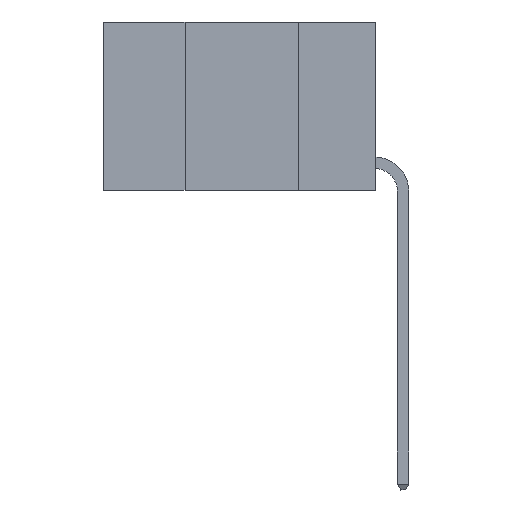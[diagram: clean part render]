
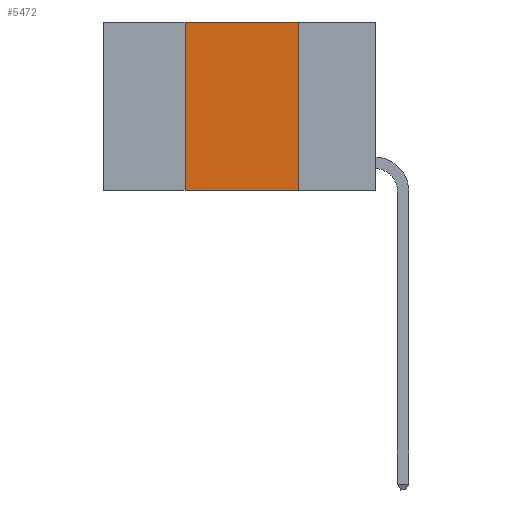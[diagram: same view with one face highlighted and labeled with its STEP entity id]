
A CAD part, left-side view. The second image highlights one B-rep face of the part: STEP entity #5472.
In plain terms, the highlighted planar face has unit normal (-1, 0, 0).
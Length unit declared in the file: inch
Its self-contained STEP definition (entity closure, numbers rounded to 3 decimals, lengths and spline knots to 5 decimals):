
#160 = ORIENTED_EDGE ( 'NONE', *, *, #1043, .F. ) ;
#1043 = EDGE_CURVE ( 'NONE', #5807, #14211, #12913, .T. ) ;
#1444 = EDGE_CURVE ( 'NONE', #13467, #11561, #16449, .T. ) ;
#3428 = CARTESIAN_POINT ( 'NONE',  ( 0., 0.6, 0. ) ) ;
#4232 = CARTESIAN_POINT ( 'NONE',  ( 0., 0.6, -0.37 ) ) ;
#4512 = DIRECTION ( 'NONE',  ( 0., 0., -1. ) ) ;
#5472 = ADVANCED_FACE ( 'NONE', ( #16959 ), #12932, .F. ) ;
#5807 = VERTEX_POINT ( 'NONE', #7192 ) ;
#5924 = AXIS2_PLACEMENT_3D ( 'NONE', #3428, #8813, #7722 ) ;
#6307 = CARTESIAN_POINT ( 'NONE',  ( 0., 0.42, 0. ) ) ;
#6615 = EDGE_CURVE ( 'NONE', #5807, #11561, #12337, .T. ) ;
#6760 = VECTOR ( 'NONE', #7875, 39.37008 ) ;
#7075 = ORIENTED_EDGE ( 'NONE', *, *, #1444, .F. ) ;
#7192 = CARTESIAN_POINT ( 'NONE',  ( 0., 0.42, -0.37 ) ) ;
#7722 = DIRECTION ( 'NONE',  ( 0., 0., -1. ) ) ;
#7875 = DIRECTION ( 'NONE',  ( 0., 0., 1. ) ) ;
#7958 = ORIENTED_EDGE ( 'NONE', *, *, #11887, .F. ) ;
#8734 = CARTESIAN_POINT ( 'NONE',  ( 0., 0.17, 0. ) ) ;
#8813 = DIRECTION ( 'NONE',  ( 1., 0., 0. ) ) ;
#10671 = CARTESIAN_POINT ( 'NONE',  ( 0., 0.17, -0.37 ) ) ;
#10825 = EDGE_LOOP ( 'NONE', ( #7075, #7958, #160, #12857 ) ) ;
#10847 = VECTOR ( 'NONE', #4512, 39.37008 ) ;
#11376 = VECTOR ( 'NONE', #15979, 39.37008 ) ;
#11561 = VERTEX_POINT ( 'NONE', #10671 ) ;
#11887 = EDGE_CURVE ( 'NONE', #14211, #13467, #16149, .T. ) ;
#12337 = LINE ( 'NONE', #4232, #14386 ) ;
#12857 = ORIENTED_EDGE ( 'NONE', *, *, #6615, .T. ) ;
#12913 = LINE ( 'NONE', #6307, #6760 ) ;
#12932 = PLANE ( 'NONE',  #5924 ) ;
#13467 = VERTEX_POINT ( 'NONE', #8734 ) ;
#13531 = CARTESIAN_POINT ( 'NONE',  ( 0., 0.42, 0. ) ) ;
#13582 = DIRECTION ( 'NONE',  ( 0., -1., 0. ) ) ;
#14211 = VERTEX_POINT ( 'NONE', #13531 ) ;
#14386 = VECTOR ( 'NONE', #13582, 39.37008 ) ;
#15979 = DIRECTION ( 'NONE',  ( 0., -1., 0. ) ) ;
#16149 = LINE ( 'NONE', #17241, #11376 ) ;
#16449 = LINE ( 'NONE', #16627, #10847 ) ;
#16627 = CARTESIAN_POINT ( 'NONE',  ( 0., 0.17, 0. ) ) ;
#16959 = FACE_OUTER_BOUND ( 'NONE', #10825, .T. ) ;
#17241 = CARTESIAN_POINT ( 'NONE',  ( 0., 0.6, 0. ) ) ;
